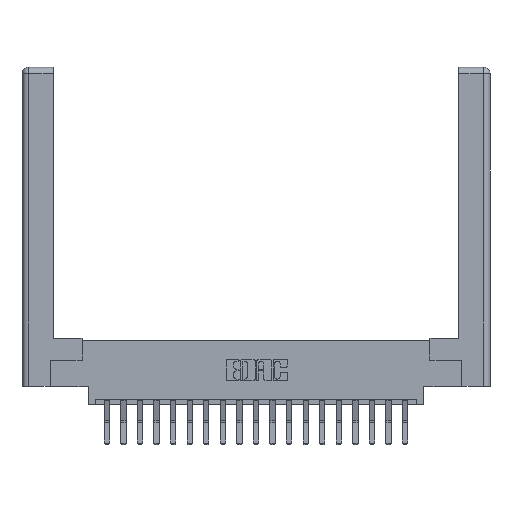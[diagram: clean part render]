
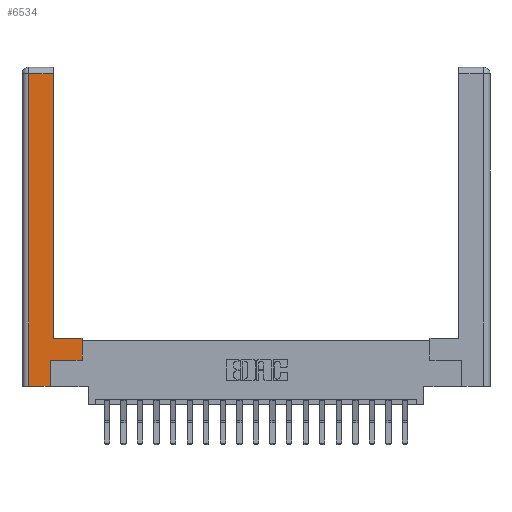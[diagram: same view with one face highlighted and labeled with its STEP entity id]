
A CAD part, top view. The second image highlights one B-rep face of the part: STEP entity #6534.
In plain terms, the highlighted planar face has unit normal (0, 0, 1).
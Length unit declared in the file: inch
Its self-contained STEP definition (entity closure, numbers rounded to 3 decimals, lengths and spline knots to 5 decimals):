
#107 = LINE ( 'NONE', #17578, #4146 ) ;
#293 = VECTOR ( 'NONE', #3757, 39.37008 ) ;
#1597 = VERTEX_POINT ( 'NONE', #20555 ) ;
#1688 = VECTOR ( 'NONE', #20570, 39.37008 ) ;
#2516 = EDGE_CURVE ( 'NONE', #7159, #18144, #8649, .T. ) ;
#2542 = VECTOR ( 'NONE', #16590, 39.37008 ) ;
#2919 = VERTEX_POINT ( 'NONE', #4181 ) ;
#3162 = CARTESIAN_POINT ( 'NONE',  ( 0.265, 0.245, 0. ) ) ;
#3334 = EDGE_LOOP ( 'NONE', ( #9906, #19397, #5083, #3670, #19067, #4961, #4870, #15582 ) ) ;
#3486 = CARTESIAN_POINT ( 'NONE',  ( 0.265, 0., 0. ) ) ;
#3670 = ORIENTED_EDGE ( 'NONE', *, *, #2516, .T. ) ;
#3725 = LINE ( 'NONE', #3162, #1688 ) ;
#3757 = DIRECTION ( 'NONE',  ( -1., 0., 0. ) ) ;
#4146 = VECTOR ( 'NONE', #8057, 39.37008 ) ;
#4181 = CARTESIAN_POINT ( 'NONE',  ( 0.295, 2.94, 0. ) ) ;
#4223 = EDGE_CURVE ( 'NONE', #7353, #6219, #107, .T. ) ;
#4391 = DIRECTION ( 'NONE',  ( -1., 0., 0. ) ) ;
#4455 = VECTOR ( 'NONE', #6828, 39.37008 ) ;
#4786 = LINE ( 'NONE', #18057, #293 ) ;
#4870 = ORIENTED_EDGE ( 'NONE', *, *, #10371, .T. ) ;
#4961 = ORIENTED_EDGE ( 'NONE', *, *, #4223, .T. ) ;
#5083 = ORIENTED_EDGE ( 'NONE', *, *, #9608, .T. ) ;
#5195 = DIRECTION ( 'NONE',  ( 0., -1., 0. ) ) ;
#5608 = VECTOR ( 'NONE', #5195, 39.37008 ) ;
#5933 = EDGE_CURVE ( 'NONE', #1597, #19522, #4786, .T. ) ;
#6219 = VERTEX_POINT ( 'NONE', #6583 ) ;
#6534 = ADVANCED_FACE ( 'NONE', ( #18456 ), #9001, .F. ) ;
#6583 = CARTESIAN_POINT ( 'NONE',  ( 0.565, 0.245, 0. ) ) ;
#6828 = DIRECTION ( 'NONE',  ( 1., 0., 0. ) ) ;
#6848 = CARTESIAN_POINT ( 'NONE',  ( 0.565, 0.45, 0. ) ) ;
#6962 = CARTESIAN_POINT ( 'NONE',  ( 0.265, 0., 0. ) ) ;
#7159 = VERTEX_POINT ( 'NONE', #19659 ) ;
#7258 = LINE ( 'NONE', #19646, #2542 ) ;
#7353 = VERTEX_POINT ( 'NONE', #18475 ) ;
#8057 = DIRECTION ( 'NONE',  ( 1., 0., 0. ) ) ;
#8624 = CARTESIAN_POINT ( 'NONE',  ( 0.295, 0.45, 0. ) ) ;
#8648 = CARTESIAN_POINT ( 'NONE',  ( 0.295, 3., 0. ) ) ;
#8649 = LINE ( 'NONE', #3486, #4455 ) ;
#8987 = EDGE_CURVE ( 'NONE', #19522, #2919, #11828, .T. ) ;
#9001 = PLANE ( 'NONE',  #13352 ) ;
#9608 = EDGE_CURVE ( 'NONE', #14519, #7159, #17259, .T. ) ;
#9906 = ORIENTED_EDGE ( 'NONE', *, *, #8987, .T. ) ;
#10371 = EDGE_CURVE ( 'NONE', #6219, #1597, #13270, .T. ) ;
#10607 = CARTESIAN_POINT ( 'NONE',  ( 0.0615, 2.94, 0. ) ) ;
#10808 = VECTOR ( 'NONE', #13450, 39.37008 ) ;
#10860 = DIRECTION ( 'NONE',  ( 0., 0., -1. ) ) ;
#11828 = LINE ( 'NONE', #8648, #10808 ) ;
#13270 = LINE ( 'NONE', #6848, #17513 ) ;
#13352 = AXIS2_PLACEMENT_3D ( 'NONE', #13888, #10860, #4391 ) ;
#13450 = DIRECTION ( 'NONE',  ( 0., 1., 0. ) ) ;
#13710 = EDGE_CURVE ( 'NONE', #18144, #7353, #3725, .T. ) ;
#13888 = CARTESIAN_POINT ( 'NONE',  ( 0., 0., 0. ) ) ;
#14399 = CARTESIAN_POINT ( 'NONE',  ( 0.0615, 0., 0. ) ) ;
#14519 = VERTEX_POINT ( 'NONE', #10607 ) ;
#14740 = EDGE_CURVE ( 'NONE', #2919, #14519, #7258, .T. ) ;
#15582 = ORIENTED_EDGE ( 'NONE', *, *, #5933, .T. ) ;
#16590 = DIRECTION ( 'NONE',  ( -1., 0., 0. ) ) ;
#17259 = LINE ( 'NONE', #14399, #5608 ) ;
#17513 = VECTOR ( 'NONE', #19480, 39.37008 ) ;
#17578 = CARTESIAN_POINT ( 'NONE',  ( 0.565, 0.245, 0. ) ) ;
#18057 = CARTESIAN_POINT ( 'NONE',  ( 0.295, 0.45, 0. ) ) ;
#18144 = VERTEX_POINT ( 'NONE', #6962 ) ;
#18456 = FACE_OUTER_BOUND ( 'NONE', #3334, .T. ) ;
#18475 = CARTESIAN_POINT ( 'NONE',  ( 0.265, 0.245, 0. ) ) ;
#19067 = ORIENTED_EDGE ( 'NONE', *, *, #13710, .T. ) ;
#19397 = ORIENTED_EDGE ( 'NONE', *, *, #14740, .T. ) ;
#19480 = DIRECTION ( 'NONE',  ( 0., 1., 0. ) ) ;
#19522 = VERTEX_POINT ( 'NONE', #8624 ) ;
#19646 = CARTESIAN_POINT ( 'NONE',  ( 0.0615, 2.94, 0. ) ) ;
#19659 = CARTESIAN_POINT ( 'NONE',  ( 0.0615, 0., 0. ) ) ;
#20555 = CARTESIAN_POINT ( 'NONE',  ( 0.565, 0.45, 0. ) ) ;
#20570 = DIRECTION ( 'NONE',  ( 0., 1., 0. ) ) ;
